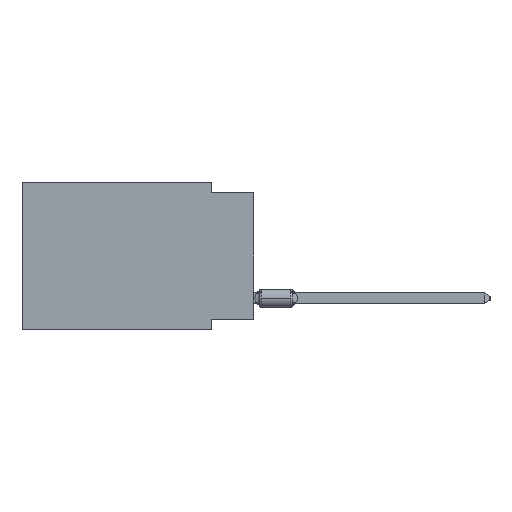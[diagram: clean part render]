
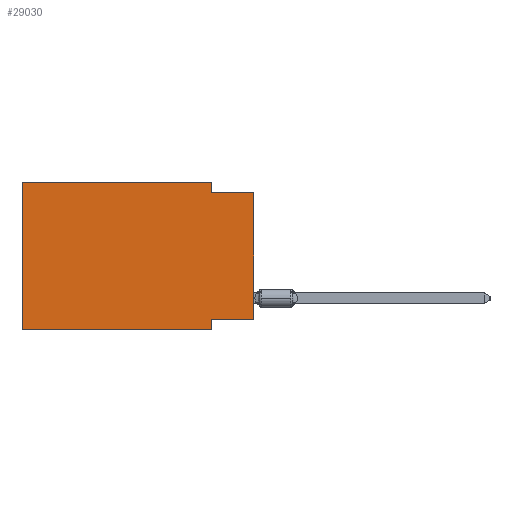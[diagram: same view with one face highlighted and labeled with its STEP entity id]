
A CAD part, left-side view. The second image highlights one B-rep face of the part: STEP entity #29030.
In plain terms, the highlighted planar face has unit normal (-1, 0, 0).
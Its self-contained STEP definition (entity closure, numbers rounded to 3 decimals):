
#820 = LINE ( 'NONE', #13547, #6189 ) ;
#1158 = CARTESIAN_POINT ( 'NONE',  ( 0., 13.97, -8.89 ) ) ;
#2080 = ORIENTED_EDGE ( 'NONE', *, *, #34732, .F. ) ;
#3736 = VERTEX_POINT ( 'NONE', #39137 ) ;
#4492 = CARTESIAN_POINT ( 'NONE',  ( 0., 2.54, 0. ) ) ;
#4884 = VERTEX_POINT ( 'NONE', #1158 ) ;
#5552 = CARTESIAN_POINT ( 'NONE',  ( 0., 2.54, -0.635 ) ) ;
#6189 = VECTOR ( 'NONE', #15702, 1000. ) ;
#6324 = CARTESIAN_POINT ( 'NONE',  ( 0., 0., -8.255 ) ) ;
#6503 = LINE ( 'NONE', #41156, #19845 ) ;
#7842 = DIRECTION ( 'NONE',  ( 0., 0., -1. ) ) ;
#9478 = ORIENTED_EDGE ( 'NONE', *, *, #13336, .F. ) ;
#9495 = VERTEX_POINT ( 'NONE', #15545 ) ;
#9695 = LINE ( 'NONE', #38906, #11903 ) ;
#10482 = VERTEX_POINT ( 'NONE', #33589 ) ;
#10975 = FACE_OUTER_BOUND ( 'NONE', #38320, .T. ) ;
#11598 = EDGE_CURVE ( 'NONE', #4884, #10482, #820, .T. ) ;
#11903 = VECTOR ( 'NONE', #15939, 1000. ) ;
#12153 = LINE ( 'NONE', #6324, #32290 ) ;
#12323 = VERTEX_POINT ( 'NONE', #5552 ) ;
#12715 = ORIENTED_EDGE ( 'NONE', *, *, #35575, .T. ) ;
#13336 = EDGE_CURVE ( 'NONE', #25140, #26886, #12153, .T. ) ;
#13547 = CARTESIAN_POINT ( 'NONE',  ( 0., 13.97, 0. ) ) ;
#13746 = LINE ( 'NONE', #32339, #31915 ) ;
#15545 = CARTESIAN_POINT ( 'NONE',  ( 0., 2.54, 0. ) ) ;
#15702 = DIRECTION ( 'NONE',  ( 0., 0., 1. ) ) ;
#15939 = DIRECTION ( 'NONE',  ( 0., -1., 0. ) ) ;
#16343 = ORIENTED_EDGE ( 'NONE', *, *, #26472, .F. ) ;
#17206 = DIRECTION ( 'NONE',  ( 0., 0., -1. ) ) ;
#18044 = DIRECTION ( 'NONE',  ( 1., 0., 0. ) ) ;
#18608 = DIRECTION ( 'NONE',  ( 0., 1., 0. ) ) ;
#18797 = DIRECTION ( 'NONE',  ( 0., -1., 0. ) ) ;
#18895 = CARTESIAN_POINT ( 'NONE',  ( 0., 0., -8.255 ) ) ;
#19845 = VECTOR ( 'NONE', #18797, 1000. ) ;
#19885 = LINE ( 'NONE', #35974, #19906 ) ;
#19906 = VECTOR ( 'NONE', #20508, 1000. ) ;
#20508 = DIRECTION ( 'NONE',  ( 0., 0., 1. ) ) ;
#21173 = CARTESIAN_POINT ( 'NONE',  ( 0., 13.97, 0. ) ) ;
#25140 = VERTEX_POINT ( 'NONE', #18895 ) ;
#26472 = EDGE_CURVE ( 'NONE', #9495, #12323, #33100, .T. ) ;
#26478 = DIRECTION ( 'NONE',  ( 0., -1., 0. ) ) ;
#26525 = VERTEX_POINT ( 'NONE', #33504 ) ;
#26563 = LINE ( 'NONE', #33051, #32507 ) ;
#26886 = VERTEX_POINT ( 'NONE', #37155 ) ;
#29030 = ADVANCED_FACE ( 'NONE', ( #10975 ), #36453, .F. ) ;
#29608 = ORIENTED_EDGE ( 'NONE', *, *, #35723, .T. ) ;
#29938 = ORIENTED_EDGE ( 'NONE', *, *, #35295, .F. ) ;
#31556 = AXIS2_PLACEMENT_3D ( 'NONE', #21173, #18044, #7842 ) ;
#31915 = VECTOR ( 'NONE', #26478, 1000. ) ;
#32290 = VECTOR ( 'NONE', #18608, 1000. ) ;
#32339 = CARTESIAN_POINT ( 'NONE',  ( 0., 0., -0.635 ) ) ;
#32507 = VECTOR ( 'NONE', #33455, 1000. ) ;
#32980 = ORIENTED_EDGE ( 'NONE', *, *, #34524, .F. ) ;
#33051 = CARTESIAN_POINT ( 'NONE',  ( 0., 2.54, -8.89 ) ) ;
#33100 = LINE ( 'NONE', #4492, #33623 ) ;
#33319 = ORIENTED_EDGE ( 'NONE', *, *, #11598, .F. ) ;
#33455 = DIRECTION ( 'NONE',  ( 0., 0., -1. ) ) ;
#33504 = CARTESIAN_POINT ( 'NONE',  ( 0., 2.54, -8.89 ) ) ;
#33589 = CARTESIAN_POINT ( 'NONE',  ( 0., 13.97, 0. ) ) ;
#33623 = VECTOR ( 'NONE', #17206, 1000. ) ;
#34524 = EDGE_CURVE ( 'NONE', #26886, #26525, #26563, .T. ) ;
#34732 = EDGE_CURVE ( 'NONE', #10482, #9495, #6503, .T. ) ;
#35295 = EDGE_CURVE ( 'NONE', #12323, #3736, #13746, .T. ) ;
#35575 = EDGE_CURVE ( 'NONE', #4884, #26525, #9695, .T. ) ;
#35723 = EDGE_CURVE ( 'NONE', #25140, #3736, #19885, .T. ) ;
#35974 = CARTESIAN_POINT ( 'NONE',  ( 0., 0., 0. ) ) ;
#36453 = PLANE ( 'NONE',  #31556 ) ;
#37155 = CARTESIAN_POINT ( 'NONE',  ( 0., 2.54, -8.255 ) ) ;
#38320 = EDGE_LOOP ( 'NONE', ( #29608, #29938, #16343, #2080, #33319, #12715, #32980, #9478 ) ) ;
#38906 = CARTESIAN_POINT ( 'NONE',  ( 0., 13.97, -8.89 ) ) ;
#39137 = CARTESIAN_POINT ( 'NONE',  ( 0., 0., -0.635 ) ) ;
#41156 = CARTESIAN_POINT ( 'NONE',  ( 0., 13.97, 0. ) ) ;
